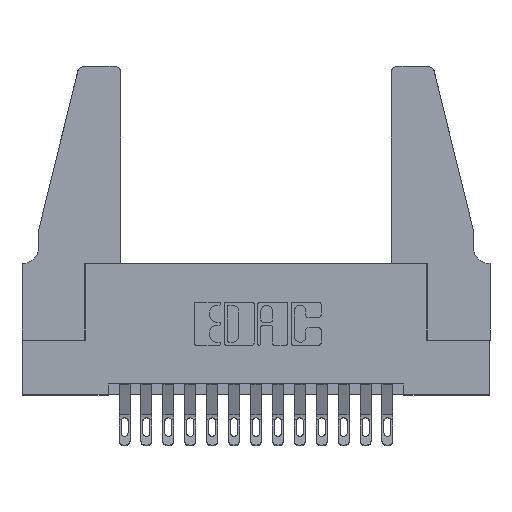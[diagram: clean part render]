
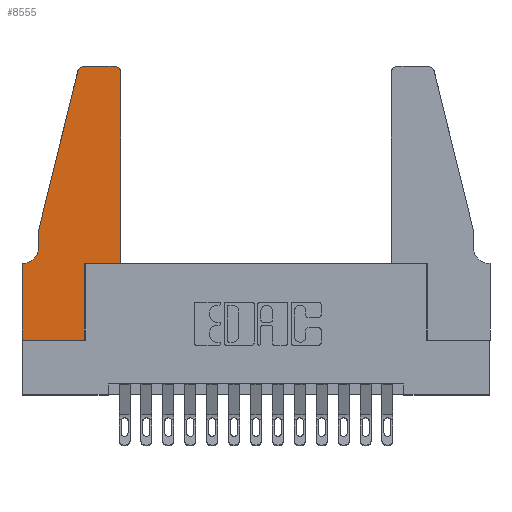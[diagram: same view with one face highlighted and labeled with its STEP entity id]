
A CAD part, top view. The second image highlights one B-rep face of the part: STEP entity #8555.
In plain terms, the highlighted planar face has unit normal (0, 0, 1).
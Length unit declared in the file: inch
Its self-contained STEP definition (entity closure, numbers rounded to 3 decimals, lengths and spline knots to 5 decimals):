
#273 = EDGE_LOOP ( 'NONE', ( #4783, #14873, #8971, #9547, #2690, #14234, #6219, #11671, #7413, #8733, #9139, #9426 ) ) ;
#348 = EDGE_CURVE ( 'NONE', #6485, #4234, #2446, .T. ) ;
#500 = CARTESIAN_POINT ( 'NONE',  ( 0.4205, 1.22, 0.37 ) ) ;
#654 = DIRECTION ( 'NONE',  ( -1., 0., 0. ) ) ;
#722 = CARTESIAN_POINT ( 'NONE',  ( 0.2605, 1.25, 0.37 ) ) ;
#812 = VECTOR ( 'NONE', #12144, 39.37008 ) ;
#923 = VERTEX_POINT ( 'NONE', #3236 ) ;
#1351 = DIRECTION ( 'NONE',  ( 1., 0., 0. ) ) ;
#1395 = EDGE_CURVE ( 'NONE', #11191, #15780, #16024, .T. ) ;
#1656 = CARTESIAN_POINT ( 'NONE',  ( 0.4505, 0.35, 0.37 ) ) ;
#1820 = DIRECTION ( 'NONE',  ( -0.239, -0.971, 0. ) ) ;
#1903 = CARTESIAN_POINT ( 'NONE',  ( 0.0755, 0.5, 0.37 ) ) ;
#1912 = CARTESIAN_POINT ( 'NONE',  ( 0.0055, 0.42, 0.37 ) ) ;
#2286 = CARTESIAN_POINT ( 'NONE',  ( 0.25487, 1.22718, 0.37 ) ) ;
#2435 = VECTOR ( 'NONE', #11788, 39.37008 ) ;
#2446 = LINE ( 'NONE', #3439, #812 ) ;
#2481 = DIRECTION ( 'NONE',  ( 0., -1., 0. ) ) ;
#2509 = VERTEX_POINT ( 'NONE', #12567 ) ;
#2544 = LINE ( 'NONE', #12763, #11139 ) ;
#2690 = ORIENTED_EDGE ( 'NONE', *, *, #6271, .T. ) ;
#2864 = CARTESIAN_POINT ( 'NONE',  ( 0.284, 1.22, 0.37 ) ) ;
#3068 = EDGE_CURVE ( 'NONE', #11697, #6583, #12600, .T. ) ;
#3192 = DIRECTION ( 'NONE',  ( 0., 0., -1. ) ) ;
#3236 = CARTESIAN_POINT ( 'NONE',  ( 0., 0.35, 0.37 ) ) ;
#3278 = EDGE_CURVE ( 'NONE', #12545, #923, #4574, .T. ) ;
#3439 = CARTESIAN_POINT ( 'NONE',  ( 0., 0., 0.37 ) ) ;
#3872 = CARTESIAN_POINT ( 'NONE',  ( 0., 0., 0.37 ) ) ;
#4175 = VECTOR ( 'NONE', #13207, 39.37008 ) ;
#4226 = CARTESIAN_POINT ( 'NONE',  ( 0.0755, 0.5, 0.37 ) ) ;
#4234 = VERTEX_POINT ( 'NONE', #10808 ) ;
#4574 = LINE ( 'NONE', #10730, #4175 ) ;
#4711 = PLANE ( 'NONE',  #6454 ) ;
#4767 = DIRECTION ( 'NONE',  ( 0., 0., 1. ) ) ;
#4774 = CARTESIAN_POINT ( 'NONE',  ( 0.284, 1.25, 0.37 ) ) ;
#4783 = ORIENTED_EDGE ( 'NONE', *, *, #7121, .T. ) ;
#5025 = DIRECTION ( 'NONE',  ( 0., 1., 0. ) ) ;
#5133 = VECTOR ( 'NONE', #1820, 39.37008 ) ;
#5355 = DIRECTION ( 'NONE',  ( 1., 0., 0. ) ) ;
#5405 = VECTOR ( 'NONE', #5355, 39.37008 ) ;
#5525 = CARTESIAN_POINT ( 'NONE',  ( 0.0755, 0.42, 0.37 ) ) ;
#5670 = DIRECTION ( 'NONE',  ( -1., 0., 0. ) ) ;
#6219 = ORIENTED_EDGE ( 'NONE', *, *, #11835, .T. ) ;
#6271 = EDGE_CURVE ( 'NONE', #12754, #12545, #6943, .T. ) ;
#6454 = AXIS2_PLACEMENT_3D ( 'NONE', #12427, #4767, #13718 ) ;
#6485 = VERTEX_POINT ( 'NONE', #3872 ) ;
#6539 = EDGE_CURVE ( 'NONE', #12182, #12754, #2544, .T. ) ;
#6583 = VERTEX_POINT ( 'NONE', #2286 ) ;
#6718 = CARTESIAN_POINT ( 'NONE',  ( 0.2865, 0.35, 0.37 ) ) ;
#6943 = CIRCLE ( 'NONE', #16461, 0.07 ) ;
#7001 = DIRECTION ( 'NONE',  ( 1., 0., 0. ) ) ;
#7121 = EDGE_CURVE ( 'NONE', #12370, #11697, #9725, .T. ) ;
#7413 = ORIENTED_EDGE ( 'NONE', *, *, #14906, .T. ) ;
#7505 = AXIS2_PLACEMENT_3D ( 'NONE', #500, #10797, #7001 ) ;
#7948 = DIRECTION ( 'NONE',  ( 0., 0., 1. ) ) ;
#8026 = LINE ( 'NONE', #6718, #2435 ) ;
#8239 = AXIS2_PLACEMENT_3D ( 'NONE', #2864, #7948, #1351 ) ;
#8453 = CIRCLE ( 'NONE', #7505, 0.03 ) ;
#8555 = ADVANCED_FACE ( 'NONE', ( #16077 ), #4711, .T. ) ;
#8716 = EDGE_CURVE ( 'NONE', #15780, #12370, #8453, .T. ) ;
#8733 = ORIENTED_EDGE ( 'NONE', *, *, #15574, .T. ) ;
#8819 = LINE ( 'NONE', #1656, #5405 ) ;
#8971 = ORIENTED_EDGE ( 'NONE', *, *, #11362, .T. ) ;
#8986 = CARTESIAN_POINT ( 'NONE',  ( 0.4505, 0.35, 0.37 ) ) ;
#9139 = ORIENTED_EDGE ( 'NONE', *, *, #1395, .T. ) ;
#9317 = VECTOR ( 'NONE', #5670, 39.37008 ) ;
#9426 = ORIENTED_EDGE ( 'NONE', *, *, #8716, .T. ) ;
#9547 = ORIENTED_EDGE ( 'NONE', *, *, #6539, .T. ) ;
#9725 = LINE ( 'NONE', #722, #9317 ) ;
#10056 = CARTESIAN_POINT ( 'NONE',  ( 0.4505, 0.35, 0.37 ) ) ;
#10130 = CARTESIAN_POINT ( 'NONE',  ( 0.4205, 1.25, 0.37 ) ) ;
#10730 = CARTESIAN_POINT ( 'NONE',  ( 0.0755, 0.35, 0.37 ) ) ;
#10797 = DIRECTION ( 'NONE',  ( 0., 0., 1. ) ) ;
#10808 = CARTESIAN_POINT ( 'NONE',  ( 0.2865, 0., 0.37 ) ) ;
#11139 = VECTOR ( 'NONE', #15354, 39.37008 ) ;
#11191 = VERTEX_POINT ( 'NONE', #8986 ) ;
#11362 = EDGE_CURVE ( 'NONE', #6583, #12182, #15756, .T. ) ;
#11456 = CARTESIAN_POINT ( 'NONE',  ( 0.0055, 0.35, 0.37 ) ) ;
#11671 = ORIENTED_EDGE ( 'NONE', *, *, #348, .T. ) ;
#11697 = VERTEX_POINT ( 'NONE', #4774 ) ;
#11788 = DIRECTION ( 'NONE',  ( 0., 1., 0. ) ) ;
#11835 = EDGE_CURVE ( 'NONE', #923, #6485, #11899, .T. ) ;
#11899 = LINE ( 'NONE', #15253, #15554 ) ;
#12144 = DIRECTION ( 'NONE',  ( 1., 0., 0. ) ) ;
#12182 = VERTEX_POINT ( 'NONE', #1903 ) ;
#12370 = VERTEX_POINT ( 'NONE', #10130 ) ;
#12427 = CARTESIAN_POINT ( 'NONE',  ( 0., 0.35, 0.37 ) ) ;
#12545 = VERTEX_POINT ( 'NONE', #11456 ) ;
#12567 = CARTESIAN_POINT ( 'NONE',  ( 0.2865, 0.35, 0.37 ) ) ;
#12600 = CIRCLE ( 'NONE', #8239, 0.03 ) ;
#12754 = VERTEX_POINT ( 'NONE', #5525 ) ;
#12763 = CARTESIAN_POINT ( 'NONE',  ( 0.0755, 0.5, 0.37 ) ) ;
#13207 = DIRECTION ( 'NONE',  ( -1., 0., 0. ) ) ;
#13718 = DIRECTION ( 'NONE',  ( 1., 0., 0. ) ) ;
#14234 = ORIENTED_EDGE ( 'NONE', *, *, #3278, .T. ) ;
#14263 = VECTOR ( 'NONE', #5025, 39.37008 ) ;
#14873 = ORIENTED_EDGE ( 'NONE', *, *, #3068, .T. ) ;
#14906 = EDGE_CURVE ( 'NONE', #4234, #2509, #8026, .T. ) ;
#15253 = CARTESIAN_POINT ( 'NONE',  ( 0., 0., 0.37 ) ) ;
#15354 = DIRECTION ( 'NONE',  ( 0., -1., 0. ) ) ;
#15554 = VECTOR ( 'NONE', #2481, 39.37008 ) ;
#15574 = EDGE_CURVE ( 'NONE', #2509, #11191, #8819, .T. ) ;
#15756 = LINE ( 'NONE', #4226, #5133 ) ;
#15780 = VERTEX_POINT ( 'NONE', #16032 ) ;
#16024 = LINE ( 'NONE', #10056, #14263 ) ;
#16032 = CARTESIAN_POINT ( 'NONE',  ( 0.4505, 1.22, 0.37 ) ) ;
#16077 = FACE_OUTER_BOUND ( 'NONE', #273, .T. ) ;
#16461 = AXIS2_PLACEMENT_3D ( 'NONE', #1912, #3192, #654 ) ;
